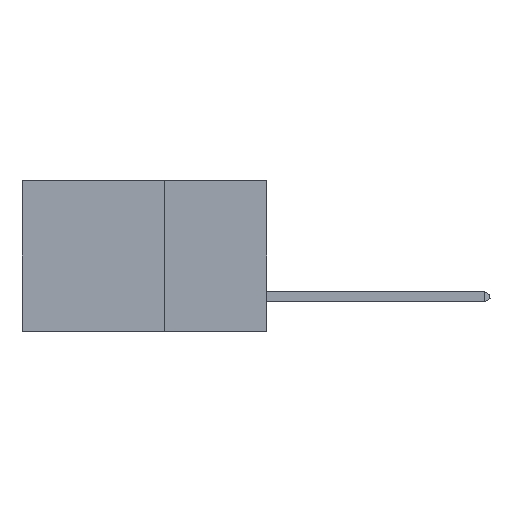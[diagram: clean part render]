
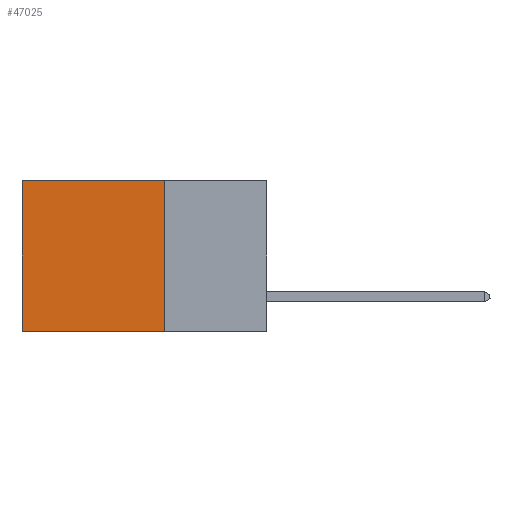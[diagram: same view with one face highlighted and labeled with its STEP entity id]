
A CAD part, left-side view. The second image highlights one B-rep face of the part: STEP entity #47025.
In plain terms, the highlighted planar face has unit normal (-1, 0, 0).
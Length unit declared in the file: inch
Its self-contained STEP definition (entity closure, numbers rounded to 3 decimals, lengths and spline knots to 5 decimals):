
#2584 = DIRECTION ( 'NONE',  ( 0., 0., -1. ) ) ;
#3583 = EDGE_CURVE ( 'NONE', #42058, #4986, #8604, .T. ) ;
#4986 = VERTEX_POINT ( 'NONE', #7528 ) ;
#7528 = CARTESIAN_POINT ( 'NONE',  ( 0.2875, 0.6, -0.37 ) ) ;
#8604 = LINE ( 'NONE', #18632, #20707 ) ;
#8608 = CARTESIAN_POINT ( 'NONE',  ( 0.2875, 0.25, -0.37 ) ) ;
#12664 = DIRECTION ( 'NONE',  ( 0., 0., -1. ) ) ;
#12703 = EDGE_CURVE ( 'NONE', #39105, #42058, #39345, .T. ) ;
#13149 = ORIENTED_EDGE ( 'NONE', *, *, #12703, .T. ) ;
#13992 = PLANE ( 'NONE',  #24336 ) ;
#14165 = VECTOR ( 'NONE', #23485, 39.37008 ) ;
#16046 = CARTESIAN_POINT ( 'NONE',  ( 0.2875, 0.25, 0. ) ) ;
#16763 = VERTEX_POINT ( 'NONE', #43980 ) ;
#18371 = CARTESIAN_POINT ( 'NONE',  ( 0.2875, 0.25, 0. ) ) ;
#18632 = CARTESIAN_POINT ( 'NONE',  ( 0.2875, 0.6, 0. ) ) ;
#20707 = VECTOR ( 'NONE', #2584, 39.37008 ) ;
#23485 = DIRECTION ( 'NONE',  ( 0., 1., 0. ) ) ;
#24336 = AXIS2_PLACEMENT_3D ( 'NONE', #25479, #32560, #40577 ) ;
#24949 = EDGE_CURVE ( 'NONE', #39105, #16763, #37179, .T. ) ;
#24955 = EDGE_CURVE ( 'NONE', #16763, #4986, #28649, .T. ) ;
#25479 = CARTESIAN_POINT ( 'NONE',  ( 0.2875, 0.25, 0. ) ) ;
#28649 = LINE ( 'NONE', #8608, #14165 ) ;
#29334 = CARTESIAN_POINT ( 'NONE',  ( 0.2875, 0.25, 0. ) ) ;
#32560 = DIRECTION ( 'NONE',  ( 1., 0., 0. ) ) ;
#33051 = DIRECTION ( 'NONE',  ( 0., 1., 0. ) ) ;
#34594 = ORIENTED_EDGE ( 'NONE', *, *, #24949, .F. ) ;
#35909 = ORIENTED_EDGE ( 'NONE', *, *, #24955, .F. ) ;
#37179 = LINE ( 'NONE', #16046, #49927 ) ;
#39105 = VERTEX_POINT ( 'NONE', #18371 ) ;
#39345 = LINE ( 'NONE', #29334, #47259 ) ;
#40577 = DIRECTION ( 'NONE',  ( 0., 0., -1. ) ) ;
#42058 = VERTEX_POINT ( 'NONE', #44309 ) ;
#43980 = CARTESIAN_POINT ( 'NONE',  ( 0.2875, 0.25, -0.37 ) ) ;
#44233 = FACE_OUTER_BOUND ( 'NONE', #45394, .T. ) ;
#44309 = CARTESIAN_POINT ( 'NONE',  ( 0.2875, 0.6, 0. ) ) ;
#45394 = EDGE_LOOP ( 'NONE', ( #48634, #35909, #34594, #13149 ) ) ;
#47025 = ADVANCED_FACE ( 'NONE', ( #44233 ), #13992, .F. ) ;
#47259 = VECTOR ( 'NONE', #33051, 39.37008 ) ;
#48634 = ORIENTED_EDGE ( 'NONE', *, *, #3583, .T. ) ;
#49927 = VECTOR ( 'NONE', #12664, 39.37008 ) ;
